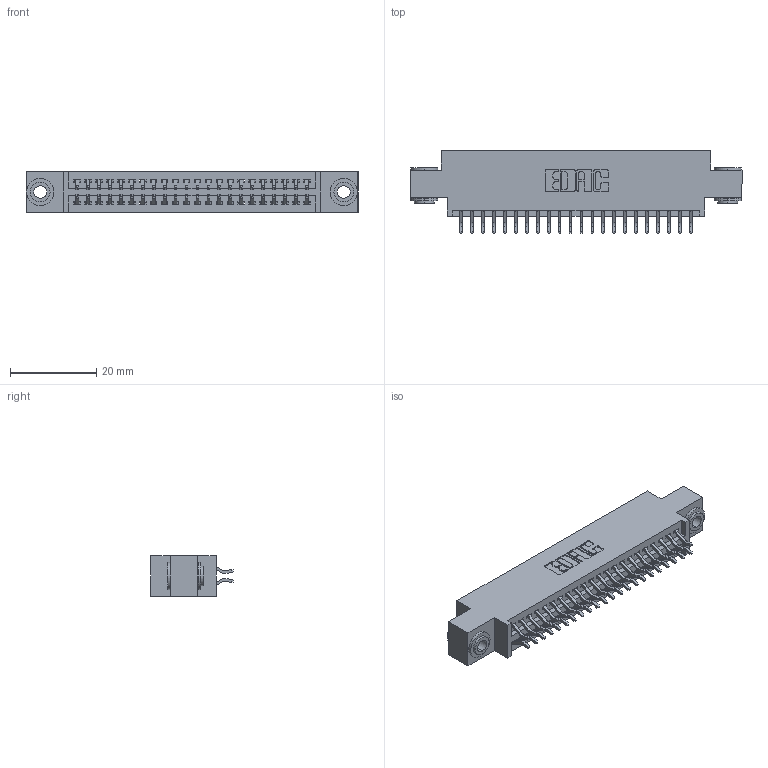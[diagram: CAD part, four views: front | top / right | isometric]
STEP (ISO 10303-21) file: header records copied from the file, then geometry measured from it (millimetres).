
FILE_DESCRIPTION (( 'STEP AP203' ), '1' );
FILE_NAME ('395-044-556-803.STEP', '2018-11-15T22:06:08', ( '' ), ( '' ), 'SwSTEP 2.0', 'SolidWorks 2016', '' );
FILE_SCHEMA (( 'CONFIG_CONTROL_DESIGN' ));
Length unit declared in the file: inch
Products named in the file (4): 345-292-001_556 Tail; 345-250-002_345-250-002-102; 395-044-556-803; 345 Part_0.170 Offset - 0.156 Dia-TH
Assembly tree (47 placements, depth 2):
  395-044-556-803
    345 Part_0.170 Offset - 0.156 Dia-TH
    345-292-001_556 Tail  x44
    345-250-002_345-250-002-102  x2
Bounding box: 77.09 x 19.24 x 9.4 mm (x, y, z)
Volume: 7207.1 mm3; surface area: 10575.8 mm2
Topology: 47 solids, 47 shells, 2632 faces, 7777 edges, 5122 vertices
Faces by surface type: plane 1722, cylinder 902, cone 8
Entity records: 20956 total; most frequent: CARTESIAN_POINT 3523, ORIENTED_EDGE 3438, DIRECTION 3149, EDGE_CURVE 1719, LINE 1467, VECTOR 1467, VERTEX_POINT 1142, AXIS2_PLACEMENT_3D 841
